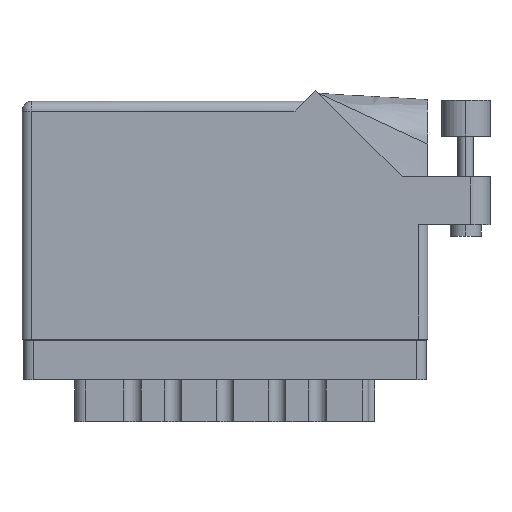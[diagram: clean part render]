
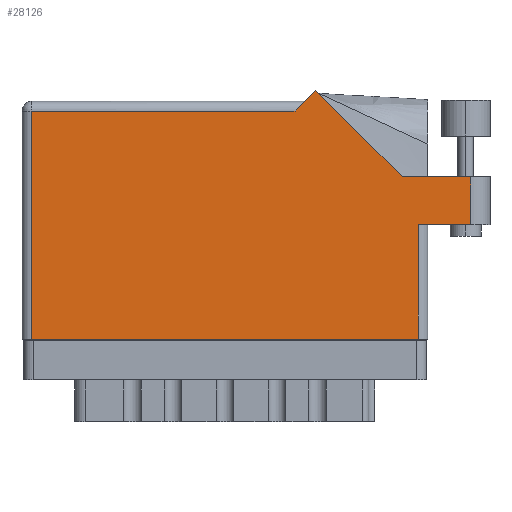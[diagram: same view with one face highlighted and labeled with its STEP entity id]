
A CAD part, front view. The second image highlights one B-rep face of the part: STEP entity #28126.
In plain terms, the highlighted face is planar.
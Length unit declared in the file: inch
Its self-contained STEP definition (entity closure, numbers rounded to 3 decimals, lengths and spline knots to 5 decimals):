
#52 = LINE ( 'NONE', #18256, #2221 ) ;
#1388 = CARTESIAN_POINT ( 'NONE',  ( 2.44642, 1.044, 0. ) ) ;
#1649 = CARTESIAN_POINT ( 'NONE',  ( 2.887, 1.044, 0. ) ) ;
#2221 = VECTOR ( 'NONE', #42536, 39.37008 ) ;
#3575 = CARTESIAN_POINT ( 'NONE',  ( 2.44642, 1.044, 0. ) ) ;
#4939 = ORIENTED_EDGE ( 'NONE', *, *, #26318, .T. ) ;
#7923 = VECTOR ( 'NONE', #34733, 39.37008 ) ;
#8428 = VERTEX_POINT ( 'NONE', #32542 ) ;
#9519 = EDGE_CURVE ( 'NONE', #8428, #34876, #36045, .T. ) ;
#10183 = CARTESIAN_POINT ( 'NONE',  ( 2.612, 0.737, 0. ) ) ;
#10214 = CARTESIAN_POINT ( 'NONE',  ( 2.55, 0.737, 0. ) ) ;
#10451 = LINE ( 'NONE', #44103, #33387 ) ;
#11041 = LINE ( 'NONE', #1649, #23088 ) ;
#12190 = CARTESIAN_POINT ( 'NONE',  ( 0., 1.53, 0. ) ) ;
#13386 = ORIENTED_EDGE ( 'NONE', *, *, #18831, .T. ) ;
#13803 = VECTOR ( 'NONE', #33359, 39.37008 ) ;
#14293 = EDGE_CURVE ( 'NONE', #34876, #41151, #10451, .T. ) ;
#14706 = VERTEX_POINT ( 'NONE', #19189 ) ;
#14949 = VECTOR ( 'NONE', #34960, 39.37008 ) ;
#15341 = VECTOR ( 'NONE', #42064, 39.37008 ) ;
#15706 = ORIENTED_EDGE ( 'NONE', *, *, #27035, .T. ) ;
#16316 = CARTESIAN_POINT ( 'NONE',  ( 1.757, 1.468, 0. ) ) ;
#16402 = VECTOR ( 'NONE', #24050, 39.37008 ) ;
#18256 = CARTESIAN_POINT ( 'NONE',  ( 2.55, 0.737, 0. ) ) ;
#18829 = EDGE_CURVE ( 'NONE', #22172, #39334, #52, .T. ) ;
#18831 = EDGE_CURVE ( 'NONE', #33153, #8428, #43052, .T. ) ;
#19189 = CARTESIAN_POINT ( 'NONE',  ( 0.062, 0., 0. ) ) ;
#21689 = CARTESIAN_POINT ( 'NONE',  ( 0., 0., 0. ) ) ;
#22172 = VERTEX_POINT ( 'NONE', #39702 ) ;
#22329 = EDGE_CURVE ( 'NONE', #32690, #33153, #23642, .T. ) ;
#23004 = FACE_OUTER_BOUND ( 'NONE', #33274, .T. ) ;
#23088 = VECTOR ( 'NONE', #28681, 39.37008 ) ;
#23642 = LINE ( 'NONE', #40447, #13803 ) ;
#24050 = DIRECTION ( 'NONE',  ( -0.707, -0.707, 0. ) ) ;
#24566 = CARTESIAN_POINT ( 'NONE',  ( 0.062, 1.468, 0. ) ) ;
#24863 = LINE ( 'NONE', #10183, #7923 ) ;
#26318 = EDGE_CURVE ( 'NONE', #41151, #14706, #31859, .T. ) ;
#26485 = CARTESIAN_POINT ( 'NONE',  ( 2.887, 1.044, 0. ) ) ;
#26832 = VERTEX_POINT ( 'NONE', #34759 ) ;
#27035 = EDGE_CURVE ( 'NONE', #26832, #32690, #11041, .T. ) ;
#28126 = ADVANCED_FACE ( 'NONE', ( #23004 ), #43470, .F. ) ;
#28171 = LINE ( 'NONE', #21689, #29263 ) ;
#28681 = DIRECTION ( 'NONE',  ( 0., 1., 0. ) ) ;
#28918 = ORIENTED_EDGE ( 'NONE', *, *, #29785, .T. ) ;
#29263 = VECTOR ( 'NONE', #42586, 39.37008 ) ;
#29785 = EDGE_CURVE ( 'NONE', #14706, #22172, #28171, .T. ) ;
#29892 = ORIENTED_EDGE ( 'NONE', *, *, #14293, .T. ) ;
#31859 = LINE ( 'NONE', #38253, #14949 ) ;
#32542 = CARTESIAN_POINT ( 'NONE',  ( 1.88971, 1.60071, 0. ) ) ;
#32690 = VERTEX_POINT ( 'NONE', #26485 ) ;
#32721 = ORIENTED_EDGE ( 'NONE', *, *, #18829, .T. ) ;
#33153 = VERTEX_POINT ( 'NONE', #1388 ) ;
#33264 = AXIS2_PLACEMENT_3D ( 'NONE', #12190, #36867, #40293 ) ;
#33274 = EDGE_LOOP ( 'NONE', ( #40942, #15706, #42956, #13386, #34476, #29892, #4939, #28918, #32721 ) ) ;
#33359 = DIRECTION ( 'NONE',  ( -1., 0., 0. ) ) ;
#33387 = VECTOR ( 'NONE', #40635, 39.37008 ) ;
#34476 = ORIENTED_EDGE ( 'NONE', *, *, #9519, .T. ) ;
#34733 = DIRECTION ( 'NONE',  ( 1., 0., 0. ) ) ;
#34759 = CARTESIAN_POINT ( 'NONE',  ( 2.887, 0.737, 0. ) ) ;
#34876 = VERTEX_POINT ( 'NONE', #16316 ) ;
#34960 = DIRECTION ( 'NONE',  ( 0., -1., 0. ) ) ;
#34982 = EDGE_CURVE ( 'NONE', #39334, #26832, #24863, .T. ) ;
#36045 = LINE ( 'NONE', #44783, #16402 ) ;
#36867 = DIRECTION ( 'NONE',  ( 0., 0., -1. ) ) ;
#38253 = CARTESIAN_POINT ( 'NONE',  ( 0.062, 0., 0. ) ) ;
#39334 = VERTEX_POINT ( 'NONE', #10214 ) ;
#39702 = CARTESIAN_POINT ( 'NONE',  ( 2.55, 0., 0. ) ) ;
#40293 = DIRECTION ( 'NONE',  ( -1., 0., 0. ) ) ;
#40447 = CARTESIAN_POINT ( 'NONE',  ( 3.012, 1.044, 0. ) ) ;
#40635 = DIRECTION ( 'NONE',  ( -1., 0., 0. ) ) ;
#40942 = ORIENTED_EDGE ( 'NONE', *, *, #34982, .T. ) ;
#41151 = VERTEX_POINT ( 'NONE', #24566 ) ;
#42064 = DIRECTION ( 'NONE',  ( -0.707, 0.707, 0. ) ) ;
#42536 = DIRECTION ( 'NONE',  ( 0., 1., 0. ) ) ;
#42586 = DIRECTION ( 'NONE',  ( 1., 0., 0. ) ) ;
#42956 = ORIENTED_EDGE ( 'NONE', *, *, #22329, .T. ) ;
#43052 = LINE ( 'NONE', #3575, #15341 ) ;
#43470 = PLANE ( 'NONE',  #33264 ) ;
#44103 = CARTESIAN_POINT ( 'NONE',  ( 0., 1.468, 0. ) ) ;
#44783 = CARTESIAN_POINT ( 'NONE',  ( 1.819, 1.53, 0. ) ) ;
